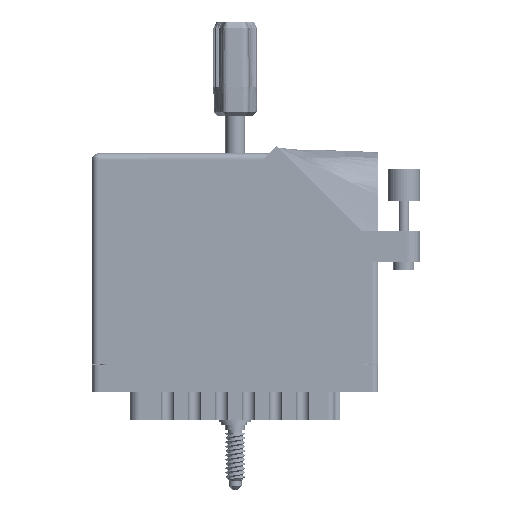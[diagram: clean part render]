
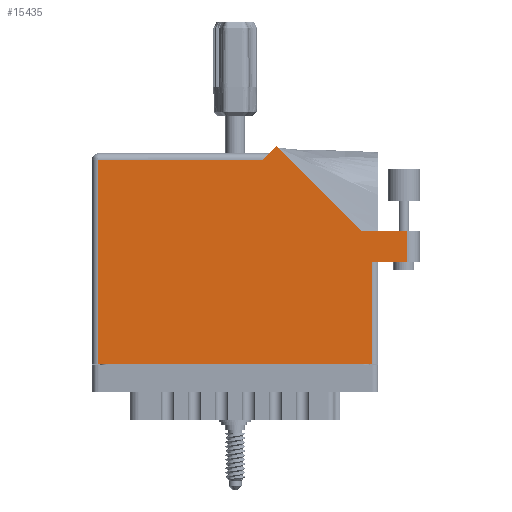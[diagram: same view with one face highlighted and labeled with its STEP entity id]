
A CAD part, front view. The second image highlights one B-rep face of the part: STEP entity #15435.
In plain terms, the highlighted face is planar.
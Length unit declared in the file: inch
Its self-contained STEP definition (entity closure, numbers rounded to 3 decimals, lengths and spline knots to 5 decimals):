
#2549 = CARTESIAN_POINT ( 'NONE',  ( 1.705, 2.03, 0. ) ) ;
#2945 = CARTESIAN_POINT ( 'NONE',  ( 2.58942, 1.287, 0. ) ) ;
#7805 = DIRECTION ( 'NONE',  ( 0., 0., -1. ) ) ;
#8658 = ORIENTED_EDGE ( 'NONE', *, *, #51871, .T. ) ;
#9514 = CARTESIAN_POINT ( 'NONE',  ( 2.693, 0.98, 0. ) ) ;
#10514 = VERTEX_POINT ( 'NONE', #72515 ) ;
#11810 = FACE_OUTER_BOUND ( 'NONE', #53641, .T. ) ;
#13162 = CARTESIAN_POINT ( 'NONE',  ( 0.062, 0., 0. ) ) ;
#15435 = ADVANCED_FACE ( 'NONE', ( #11810 ), #75834, .F. ) ;
#16556 = VERTEX_POINT ( 'NONE', #54090 ) ;
#17372 = VECTOR ( 'NONE', #39719, 39.37008 ) ;
#17798 = VERTEX_POINT ( 'NONE', #22698 ) ;
#17864 = CARTESIAN_POINT ( 'NONE',  ( 0., 0., 0. ) ) ;
#19932 = DIRECTION ( 'NONE',  ( -0.707, -0.707, 0. ) ) ;
#21261 = VERTEX_POINT ( 'NONE', #41710 ) ;
#21329 = VECTOR ( 'NONE', #104234, 39.37008 ) ;
#22698 = CARTESIAN_POINT ( 'NONE',  ( 0.062, 1.968, 0. ) ) ;
#22841 = EDGE_CURVE ( 'NONE', #17798, #42795, #100741, .T. ) ;
#28565 = CARTESIAN_POINT ( 'NONE',  ( 1.77571, 2.10071, 0. ) ) ;
#30908 = EDGE_CURVE ( 'NONE', #91516, #10514, #58114, .T. ) ;
#33494 = VECTOR ( 'NONE', #58583, 39.37008 ) ;
#38463 = VECTOR ( 'NONE', #102149, 39.37008 ) ;
#39235 = ORIENTED_EDGE ( 'NONE', *, *, #50611, .T. ) ;
#39719 = DIRECTION ( 'NONE',  ( -1., 0., 0. ) ) ;
#41710 = CARTESIAN_POINT ( 'NONE',  ( 2.693, 0.98, 0. ) ) ;
#42795 = VERTEX_POINT ( 'NONE', #84009 ) ;
#44165 = VECTOR ( 'NONE', #19932, 39.37008 ) ;
#45170 = ORIENTED_EDGE ( 'NONE', *, *, #22841, .T. ) ;
#48833 = ORIENTED_EDGE ( 'NONE', *, *, #30908, .T. ) ;
#50611 = EDGE_CURVE ( 'NONE', #63386, #16556, #50698, .T. ) ;
#50698 = LINE ( 'NONE', #2549, #44165 ) ;
#51871 = EDGE_CURVE ( 'NONE', #84796, #63386, #75529, .T. ) ;
#52264 = EDGE_CURVE ( 'NONE', #68461, #21261, #86021, .T. ) ;
#53641 = EDGE_LOOP ( 'NONE', ( #63589, #48833, #86410, #8658, #39235, #62587, #45170, #80255, #63643 ) ) ;
#54090 = CARTESIAN_POINT ( 'NONE',  ( 1.643, 1.968, 0. ) ) ;
#55134 = CARTESIAN_POINT ( 'NONE',  ( 3.155, 1.287, 0. ) ) ;
#55282 = CARTESIAN_POINT ( 'NONE',  ( 2.755, 0.98, 0. ) ) ;
#56959 = VECTOR ( 'NONE', #76814, 39.37008 ) ;
#58114 = LINE ( 'NONE', #93994, #105586 ) ;
#58291 = AXIS2_PLACEMENT_3D ( 'NONE', #76881, #7805, #58815 ) ;
#58583 = DIRECTION ( 'NONE',  ( 1., 0., 0. ) ) ;
#58815 = DIRECTION ( 'NONE',  ( -1., 0., 0. ) ) ;
#60840 = EDGE_CURVE ( 'NONE', #42795, #68461, #67458, .T. ) ;
#62081 = CARTESIAN_POINT ( 'NONE',  ( 3.03, 0.98, 0. ) ) ;
#62587 = ORIENTED_EDGE ( 'NONE', *, *, #72301, .T. ) ;
#63386 = VERTEX_POINT ( 'NONE', #28565 ) ;
#63483 = EDGE_CURVE ( 'NONE', #10514, #84796, #91390, .T. ) ;
#63589 = ORIENTED_EDGE ( 'NONE', *, *, #98046, .T. ) ;
#63643 = ORIENTED_EDGE ( 'NONE', *, *, #52264, .T. ) ;
#66550 = LINE ( 'NONE', #55282, #33494 ) ;
#67411 = DIRECTION ( 'NONE',  ( 0., 1., 0. ) ) ;
#67458 = LINE ( 'NONE', #17864, #38463 ) ;
#68461 = VERTEX_POINT ( 'NONE', #98957 ) ;
#72301 = EDGE_CURVE ( 'NONE', #16556, #17798, #94045, .T. ) ;
#72515 = CARTESIAN_POINT ( 'NONE',  ( 3.03, 1.287, 0. ) ) ;
#75479 = DIRECTION ( 'NONE',  ( -1., 0., 0. ) ) ;
#75529 = LINE ( 'NONE', #2945, #21329 ) ;
#75834 = PLANE ( 'NONE',  #58291 ) ;
#76814 = DIRECTION ( 'NONE',  ( 0., 1., 0. ) ) ;
#76881 = CARTESIAN_POINT ( 'NONE',  ( 0., 2.03, 0. ) ) ;
#80255 = ORIENTED_EDGE ( 'NONE', *, *, #60840, .T. ) ;
#84009 = CARTESIAN_POINT ( 'NONE',  ( 0.062, 0., 0. ) ) ;
#84796 = VERTEX_POINT ( 'NONE', #100161 ) ;
#86021 = LINE ( 'NONE', #9514, #56959 ) ;
#86410 = ORIENTED_EDGE ( 'NONE', *, *, #63483, .T. ) ;
#91390 = LINE ( 'NONE', #55134, #104629 ) ;
#91516 = VERTEX_POINT ( 'NONE', #62081 ) ;
#92742 = VECTOR ( 'NONE', #106691, 39.37008 ) ;
#93994 = CARTESIAN_POINT ( 'NONE',  ( 3.03, 1.287, 0. ) ) ;
#94045 = LINE ( 'NONE', #107675, #17372 ) ;
#98046 = EDGE_CURVE ( 'NONE', #21261, #91516, #66550, .T. ) ;
#98957 = CARTESIAN_POINT ( 'NONE',  ( 2.693, 0., 0. ) ) ;
#100161 = CARTESIAN_POINT ( 'NONE',  ( 2.58942, 1.287, 0. ) ) ;
#100741 = LINE ( 'NONE', #13162, #92742 ) ;
#102149 = DIRECTION ( 'NONE',  ( 1., 0., 0. ) ) ;
#104234 = DIRECTION ( 'NONE',  ( -0.707, 0.707, 0. ) ) ;
#104629 = VECTOR ( 'NONE', #75479, 39.37008 ) ;
#105586 = VECTOR ( 'NONE', #67411, 39.37008 ) ;
#106691 = DIRECTION ( 'NONE',  ( 0., -1., 0. ) ) ;
#107675 = CARTESIAN_POINT ( 'NONE',  ( 0., 1.968, 0. ) ) ;
